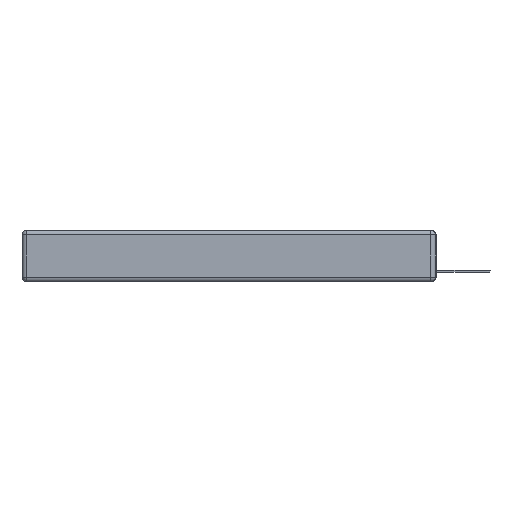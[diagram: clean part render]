
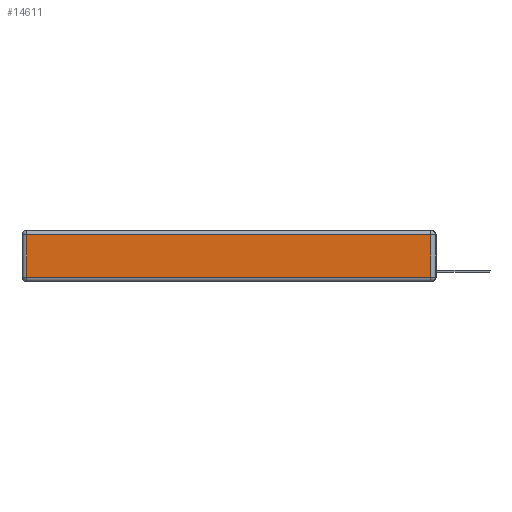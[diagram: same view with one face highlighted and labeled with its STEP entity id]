
A CAD part, left-side view. The second image highlights one B-rep face of the part: STEP entity #14611.
In plain terms, the highlighted planar face has unit normal (-1, 0, 0).
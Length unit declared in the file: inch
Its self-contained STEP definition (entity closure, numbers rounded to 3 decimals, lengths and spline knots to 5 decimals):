
#146 = DIRECTION ( 'NONE',  ( -1., 0., 0. ) ) ;
#1502 = AXIS2_PLACEMENT_3D ( 'NONE', #4907, #146, #5220 ) ;
#2364 = LINE ( 'NONE', #13245, #8433 ) ;
#4000 = LINE ( 'NONE', #13428, #8974 ) ;
#4104 = EDGE_CURVE ( 'NONE', #6220, #6223, #2364, .T. ) ;
#4252 = VECTOR ( 'NONE', #5037, 39.37008 ) ;
#4907 = CARTESIAN_POINT ( 'NONE',  ( 0., 0., -0.343 ) ) ;
#5037 = DIRECTION ( 'NONE',  ( 0., 0., 1. ) ) ;
#5220 = DIRECTION ( 'NONE',  ( 0., 0., 1. ) ) ;
#5417 = CARTESIAN_POINT ( 'NONE',  ( 0., 2.72, -0.03 ) ) ;
#5676 = EDGE_CURVE ( 'NONE', #14816, #20302, #11279, .T. ) ;
#6220 = VERTEX_POINT ( 'NONE', #6973 ) ;
#6223 = VERTEX_POINT ( 'NONE', #5417 ) ;
#6973 = CARTESIAN_POINT ( 'NONE',  ( 0., 0.03, -0.03 ) ) ;
#7379 = EDGE_CURVE ( 'NONE', #20302, #6220, #14646, .T. ) ;
#8433 = VECTOR ( 'NONE', #19781, 39.37008 ) ;
#8565 = CARTESIAN_POINT ( 'NONE',  ( 0., 0.03, -0.343 ) ) ;
#8772 = ORIENTED_EDGE ( 'NONE', *, *, #17461, .T. ) ;
#8974 = VECTOR ( 'NONE', #14958, 39.37008 ) ;
#9722 = DIRECTION ( 'NONE',  ( 0., -1., 0. ) ) ;
#9989 = FACE_OUTER_BOUND ( 'NONE', #18235, .T. ) ;
#10387 = CARTESIAN_POINT ( 'NONE',  ( 0., 2.72, -0.313 ) ) ;
#11279 = LINE ( 'NONE', #19178, #15472 ) ;
#12616 = ORIENTED_EDGE ( 'NONE', *, *, #4104, .T. ) ;
#13245 = CARTESIAN_POINT ( 'NONE',  ( 0., 2.75, -0.03 ) ) ;
#13428 = CARTESIAN_POINT ( 'NONE',  ( 0., 2.72, -0.343 ) ) ;
#14611 = ADVANCED_FACE ( 'NONE', ( #9989 ), #16158, .T. ) ;
#14646 = LINE ( 'NONE', #8565, #4252 ) ;
#14816 = VERTEX_POINT ( 'NONE', #10387 ) ;
#14958 = DIRECTION ( 'NONE',  ( 0., 0., -1. ) ) ;
#15472 = VECTOR ( 'NONE', #9722, 39.37008 ) ;
#15943 = ORIENTED_EDGE ( 'NONE', *, *, #5676, .T. ) ;
#16158 = PLANE ( 'NONE',  #1502 ) ;
#16240 = CARTESIAN_POINT ( 'NONE',  ( 0., 0.03, -0.313 ) ) ;
#17461 = EDGE_CURVE ( 'NONE', #6223, #14816, #4000, .T. ) ;
#18235 = EDGE_LOOP ( 'NONE', ( #15943, #20226, #12616, #8772 ) ) ;
#19178 = CARTESIAN_POINT ( 'NONE',  ( 0., 0., -0.313 ) ) ;
#19781 = DIRECTION ( 'NONE',  ( 0., 1., 0. ) ) ;
#20226 = ORIENTED_EDGE ( 'NONE', *, *, #7379, .T. ) ;
#20302 = VERTEX_POINT ( 'NONE', #16240 ) ;
